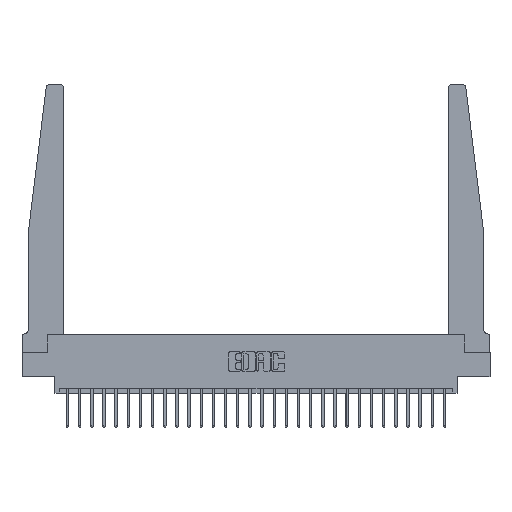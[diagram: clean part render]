
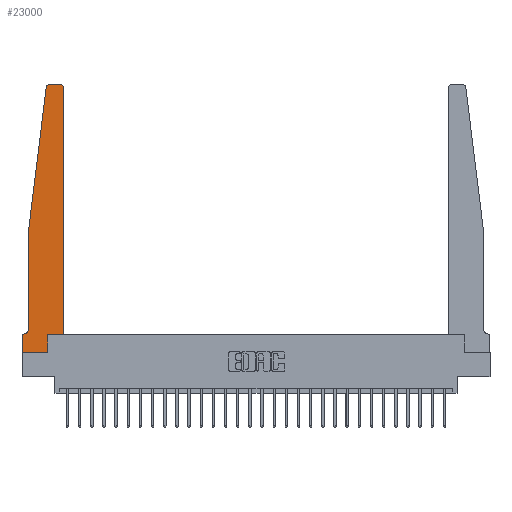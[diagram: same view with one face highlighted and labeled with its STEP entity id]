
A CAD part, top view. The second image highlights one B-rep face of the part: STEP entity #23000.
In plain terms, the highlighted planar face has unit normal (0, 0, 1).
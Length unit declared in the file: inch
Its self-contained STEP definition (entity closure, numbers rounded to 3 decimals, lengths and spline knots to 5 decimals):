
#345 = ORIENTED_EDGE ( 'NONE', *, *, #18076, .T. ) ;
#478 = VERTEX_POINT ( 'NONE', #6056 ) ;
#798 = CARTESIAN_POINT ( 'NONE',  ( 0., 0., 0.37 ) ) ;
#1179 = CIRCLE ( 'NONE', #11718, 0.03 ) ;
#1653 = EDGE_CURVE ( 'NONE', #9371, #14974, #3325, .T. ) ;
#1683 = VERTEX_POINT ( 'NONE', #3730 ) ;
#1780 = LINE ( 'NONE', #18536, #23430 ) ;
#2422 = VECTOR ( 'NONE', #14241, 39.37008 ) ;
#3069 = CARTESIAN_POINT ( 'NONE',  ( 0.395, 2.75, 0.37 ) ) ;
#3087 = LINE ( 'NONE', #16264, #2422 ) ;
#3298 = CARTESIAN_POINT ( 'NONE',  ( 0.065, 0.2375, 0.37 ) ) ;
#3325 = LINE ( 'NONE', #16280, #19410 ) ;
#3679 = FACE_OUTER_BOUND ( 'NONE', #25058, .T. ) ;
#3730 = CARTESIAN_POINT ( 'NONE',  ( 0.27653, 2.75, 0.37 ) ) ;
#4234 = DIRECTION ( 'NONE',  ( 0., 1., 0. ) ) ;
#4605 = EDGE_CURVE ( 'NONE', #23097, #1683, #22191, .T. ) ;
#4840 = DIRECTION ( 'NONE',  ( 0., 0., 1. ) ) ;
#5846 = DIRECTION ( 'NONE',  ( 0., 0., -1. ) ) ;
#5944 = VERTEX_POINT ( 'NONE', #3298 ) ;
#6056 = CARTESIAN_POINT ( 'NONE',  ( 0.425, 2.72, 0.37 ) ) ;
#6078 = VERTEX_POINT ( 'NONE', #9976 ) ;
#6193 = VECTOR ( 'NONE', #17017, 39.37008 ) ;
#6257 = CARTESIAN_POINT ( 'NONE',  ( 0.27653, 2.72, 0.37 ) ) ;
#6684 = EDGE_CURVE ( 'NONE', #478, #23097, #1179, .T. ) ;
#8051 = VERTEX_POINT ( 'NONE', #12368 ) ;
#8124 = DIRECTION ( 'NONE',  ( 0., 0., 1. ) ) ;
#8359 = DIRECTION ( 'NONE',  ( 1., 0., 0. ) ) ;
#8372 = VECTOR ( 'NONE', #4234, 39.37008 ) ;
#8660 = EDGE_CURVE ( 'NONE', #6078, #478, #1780, .T. ) ;
#8915 = LINE ( 'NONE', #18493, #24890 ) ;
#9090 = EDGE_CURVE ( 'NONE', #8051, #14560, #3087, .T. ) ;
#9371 = VERTEX_POINT ( 'NONE', #19476 ) ;
#9490 = AXIS2_PLACEMENT_3D ( 'NONE', #11134, #4840, #19501 ) ;
#9673 = EDGE_CURVE ( 'NONE', #5944, #26846, #22724, .T. ) ;
#9831 = EDGE_CURVE ( 'NONE', #20761, #10113, #20138, .T. ) ;
#9976 = CARTESIAN_POINT ( 'NONE',  ( 0.425, 0.18, 0.37 ) ) ;
#10095 = CARTESIAN_POINT ( 'NONE',  ( 0.065, 1.25, 0.37 ) ) ;
#10113 = VERTEX_POINT ( 'NONE', #15556 ) ;
#11006 = CARTESIAN_POINT ( 'NONE',  ( 0.065, 1.25, 0.37 ) ) ;
#11134 = CARTESIAN_POINT ( 'NONE',  ( 0., 0.1875, 0.37 ) ) ;
#11718 = AXIS2_PLACEMENT_3D ( 'NONE', #20631, #8124, #22691 ) ;
#12368 = CARTESIAN_POINT ( 'NONE',  ( 0., 0.1875, 0.37 ) ) ;
#12654 = CARTESIAN_POINT ( 'NONE',  ( 0.2605, 0.18, 0.37 ) ) ;
#12938 = ORIENTED_EDGE ( 'NONE', *, *, #17786, .T. ) ;
#13957 = VECTOR ( 'NONE', #26734, 39.37008 ) ;
#14241 = DIRECTION ( 'NONE',  ( 0., -1., 0. ) ) ;
#14464 = ORIENTED_EDGE ( 'NONE', *, *, #19462, .T. ) ;
#14487 = ORIENTED_EDGE ( 'NONE', *, *, #22282, .T. ) ;
#14560 = VERTEX_POINT ( 'NONE', #17794 ) ;
#14838 = CARTESIAN_POINT ( 'NONE',  ( 0.015, 0.1875, 0.37 ) ) ;
#14974 = VERTEX_POINT ( 'NONE', #11006 ) ;
#15429 = AXIS2_PLACEMENT_3D ( 'NONE', #18386, #5846, #20490 ) ;
#15556 = CARTESIAN_POINT ( 'NONE',  ( 0.2605, 0.18, 0.37 ) ) ;
#16264 = CARTESIAN_POINT ( 'NONE',  ( 0., 0., 0.37 ) ) ;
#16265 = DIRECTION ( 'NONE',  ( -1., 0., 0. ) ) ;
#16280 = CARTESIAN_POINT ( 'NONE',  ( 0.065, 1.25, 0.37 ) ) ;
#16444 = DIRECTION ( 'NONE',  ( 1., 0., 0. ) ) ;
#16563 = DIRECTION ( 'NONE',  ( 0., 1., 0. ) ) ;
#16846 = CIRCLE ( 'NONE', #25535, 0.03 ) ;
#16940 = ORIENTED_EDGE ( 'NONE', *, *, #23428, .T. ) ;
#17017 = DIRECTION ( 'NONE',  ( -1., 0., 0. ) ) ;
#17113 = ORIENTED_EDGE ( 'NONE', *, *, #6684, .T. ) ;
#17395 = VECTOR ( 'NONE', #23914, 39.37008 ) ;
#17786 = EDGE_CURVE ( 'NONE', #10113, #6078, #8915, .T. ) ;
#17794 = CARTESIAN_POINT ( 'NONE',  ( 0., 0., 0.37 ) ) ;
#17826 = ORIENTED_EDGE ( 'NONE', *, *, #4605, .T. ) ;
#18076 = EDGE_CURVE ( 'NONE', #14560, #20761, #22913, .T. ) ;
#18386 = CARTESIAN_POINT ( 'NONE',  ( 0.015, 0.2375, 0.37 ) ) ;
#18493 = CARTESIAN_POINT ( 'NONE',  ( 0.425, 0.18, 0.37 ) ) ;
#18536 = CARTESIAN_POINT ( 'NONE',  ( 0.425, 0.18, 0.37 ) ) ;
#18612 = VECTOR ( 'NONE', #16265, 39.37008 ) ;
#19304 = ORIENTED_EDGE ( 'NONE', *, *, #8660, .T. ) ;
#19410 = VECTOR ( 'NONE', #26585, 39.37008 ) ;
#19462 = EDGE_CURVE ( 'NONE', #26846, #8051, #24136, .T. ) ;
#19476 = CARTESIAN_POINT ( 'NONE',  ( 0.24675, 2.72367, 0.37 ) ) ;
#19501 = DIRECTION ( 'NONE',  ( 1., 0., 0. ) ) ;
#20138 = LINE ( 'NONE', #12654, #8372 ) ;
#20325 = ORIENTED_EDGE ( 'NONE', *, *, #9090, .T. ) ;
#20490 = DIRECTION ( 'NONE',  ( -1., 0., 0. ) ) ;
#20630 = ORIENTED_EDGE ( 'NONE', *, *, #9673, .T. ) ;
#20631 = CARTESIAN_POINT ( 'NONE',  ( 0.395, 2.72, 0.37 ) ) ;
#20761 = VERTEX_POINT ( 'NONE', #25980 ) ;
#20880 = DIRECTION ( 'NONE',  ( 0., 0., 1. ) ) ;
#22191 = LINE ( 'NONE', #25264, #6193 ) ;
#22282 = EDGE_CURVE ( 'NONE', #14974, #5944, #25005, .T. ) ;
#22691 = DIRECTION ( 'NONE',  ( 1., 0., 0. ) ) ;
#22724 = CIRCLE ( 'NONE', #15429, 0.05 ) ;
#22913 = LINE ( 'NONE', #798, #17395 ) ;
#23000 = ADVANCED_FACE ( 'NONE', ( #3679 ), #23585, .T. ) ;
#23097 = VERTEX_POINT ( 'NONE', #3069 ) ;
#23137 = ORIENTED_EDGE ( 'NONE', *, *, #1653, .T. ) ;
#23428 = EDGE_CURVE ( 'NONE', #1683, #9371, #16846, .T. ) ;
#23430 = VECTOR ( 'NONE', #16563, 39.37008 ) ;
#23585 = PLANE ( 'NONE',  #9490 ) ;
#23914 = DIRECTION ( 'NONE',  ( 1., 0., 0. ) ) ;
#24136 = LINE ( 'NONE', #26572, #18612 ) ;
#24890 = VECTOR ( 'NONE', #16444, 39.37008 ) ;
#25005 = LINE ( 'NONE', #10095, #13957 ) ;
#25058 = EDGE_LOOP ( 'NONE', ( #17826, #16940, #23137, #14487, #20630, #14464, #20325, #345, #26058, #12938, #19304, #17113 ) ) ;
#25264 = CARTESIAN_POINT ( 'NONE',  ( 0.25, 2.75, 0.37 ) ) ;
#25535 = AXIS2_PLACEMENT_3D ( 'NONE', #6257, #20880, #8359 ) ;
#25980 = CARTESIAN_POINT ( 'NONE',  ( 0.2605, 0., 0.37 ) ) ;
#26058 = ORIENTED_EDGE ( 'NONE', *, *, #9831, .T. ) ;
#26572 = CARTESIAN_POINT ( 'NONE',  ( 0.065, 0.1875, 0.37 ) ) ;
#26585 = DIRECTION ( 'NONE',  ( -0.122, -0.992, 0. ) ) ;
#26734 = DIRECTION ( 'NONE',  ( 0., -1., 0. ) ) ;
#26846 = VERTEX_POINT ( 'NONE', #14838 ) ;
